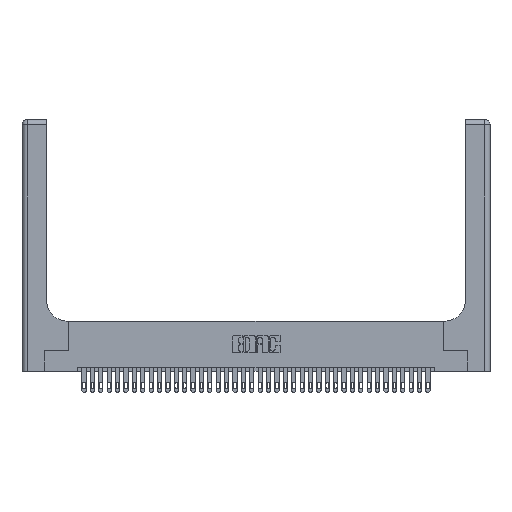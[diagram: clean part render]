
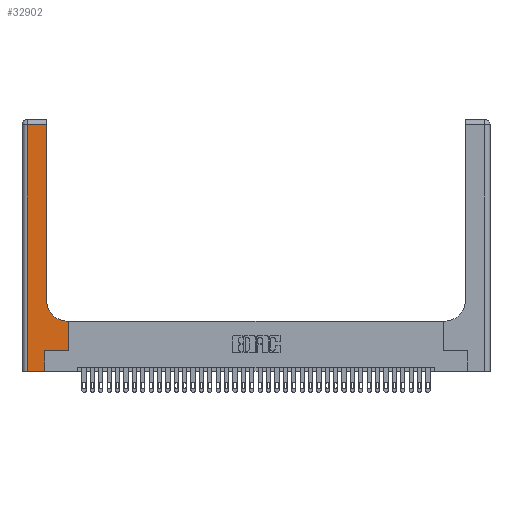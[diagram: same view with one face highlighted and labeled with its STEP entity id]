
A CAD part, top view. The second image highlights one B-rep face of the part: STEP entity #32902.
In plain terms, the highlighted planar face has unit normal (0, 0, 1).
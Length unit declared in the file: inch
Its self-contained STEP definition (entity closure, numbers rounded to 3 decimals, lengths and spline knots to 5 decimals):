
#487 = EDGE_CURVE ( 'NONE', #10428, #34353, #5170, .T. ) ;
#546 = CARTESIAN_POINT ( 'NONE',  ( 0.5585, 0.6, 0.37 ) ) ;
#2104 = CARTESIAN_POINT ( 'NONE',  ( 0.2915, 3., 0.37 ) ) ;
#2393 = ORIENTED_EDGE ( 'NONE', *, *, #11467, .T. ) ;
#2413 = CARTESIAN_POINT ( 'NONE',  ( 0.06, 3., 0.37 ) ) ;
#2970 = ORIENTED_EDGE ( 'NONE', *, *, #487, .T. ) ;
#3440 = VERTEX_POINT ( 'NONE', #29615 ) ;
#3580 = LINE ( 'NONE', #2104, #23335 ) ;
#5170 = LINE ( 'NONE', #30197, #10217 ) ;
#5419 = DIRECTION ( 'NONE',  ( -1., 0., 0. ) ) ;
#5505 = DIRECTION ( 'NONE',  ( -1., 0., 0. ) ) ;
#7911 = AXIS2_PLACEMENT_3D ( 'NONE', #28503, #28618, #5505 ) ;
#8545 = VECTOR ( 'NONE', #29272, 39.37008 ) ;
#9003 = ORIENTED_EDGE ( 'NONE', *, *, #17756, .T. ) ;
#9184 = DIRECTION ( 'NONE',  ( 1., 0., 0. ) ) ;
#9576 = ORIENTED_EDGE ( 'NONE', *, *, #9922, .T. ) ;
#9711 = EDGE_CURVE ( 'NONE', #27332, #13544, #22761, .T. ) ;
#9922 = EDGE_CURVE ( 'NONE', #34353, #3440, #23242, .T. ) ;
#10217 = VECTOR ( 'NONE', #21434, 39.37008 ) ;
#10428 = VERTEX_POINT ( 'NONE', #35386 ) ;
#10843 = VERTEX_POINT ( 'NONE', #28950 ) ;
#11359 = EDGE_CURVE ( 'NONE', #13544, #36346, #17511, .T. ) ;
#11467 = EDGE_CURVE ( 'NONE', #3440, #10843, #12934, .T. ) ;
#11985 = VERTEX_POINT ( 'NONE', #13174 ) ;
#12031 = VECTOR ( 'NONE', #14788, 39.37008 ) ;
#12079 = LINE ( 'NONE', #25442, #28228 ) ;
#12096 = ORIENTED_EDGE ( 'NONE', *, *, #37684, .T. ) ;
#12724 = ORIENTED_EDGE ( 'NONE', *, *, #9711, .T. ) ;
#12739 = CARTESIAN_POINT ( 'NONE',  ( 0.06, 2.94, 0.37 ) ) ;
#12934 = LINE ( 'NONE', #34843, #12031 ) ;
#13174 = CARTESIAN_POINT ( 'NONE',  ( 0.2915, 0.85, 0.37 ) ) ;
#13365 = EDGE_CURVE ( 'NONE', #11985, #10428, #3580, .T. ) ;
#13544 = VERTEX_POINT ( 'NONE', #546 ) ;
#14788 = DIRECTION ( 'NONE',  ( 1., 0., 0. ) ) ;
#17511 = LINE ( 'NONE', #29378, #19340 ) ;
#17756 = EDGE_CURVE ( 'NONE', #36346, #11985, #18513, .T. ) ;
#18512 = CARTESIAN_POINT ( 'NONE',  ( 0.269, 0.25, 0.37 ) ) ;
#18513 = CIRCLE ( 'NONE', #22358, 0.25 ) ;
#19340 = VECTOR ( 'NONE', #5419, 39.37008 ) ;
#19390 = LINE ( 'NONE', #18512, #28598 ) ;
#19884 = ORIENTED_EDGE ( 'NONE', *, *, #37550, .T. ) ;
#19935 = DIRECTION ( 'NONE',  ( 0., 1., 0. ) ) ;
#20149 = CARTESIAN_POINT ( 'NONE',  ( 0.5415, 0.6, 0.37 ) ) ;
#20582 = CARTESIAN_POINT ( 'NONE',  ( 0.5585, 0.25, 0.37 ) ) ;
#21181 = CARTESIAN_POINT ( 'NONE',  ( 0.269, 0.25, 0.37 ) ) ;
#21434 = DIRECTION ( 'NONE',  ( -1., 0., 0. ) ) ;
#21759 = ORIENTED_EDGE ( 'NONE', *, *, #13365, .T. ) ;
#21878 = FACE_OUTER_BOUND ( 'NONE', #36560, .T. ) ;
#22358 = AXIS2_PLACEMENT_3D ( 'NONE', #29987, #32949, #9184 ) ;
#22761 = LINE ( 'NONE', #23166, #30592 ) ;
#23166 = CARTESIAN_POINT ( 'NONE',  ( 0.5585, 0.25, 0.37 ) ) ;
#23242 = LINE ( 'NONE', #2413, #8545 ) ;
#23335 = VECTOR ( 'NONE', #19935, 39.37008 ) ;
#25442 = CARTESIAN_POINT ( 'NONE',  ( 0.269, 0., 0.37 ) ) ;
#27332 = VERTEX_POINT ( 'NONE', #20582 ) ;
#27481 = ORIENTED_EDGE ( 'NONE', *, *, #11359, .T. ) ;
#28096 = PLANE ( 'NONE',  #7911 ) ;
#28228 = VECTOR ( 'NONE', #31104, 39.37008 ) ;
#28503 = CARTESIAN_POINT ( 'NONE',  ( 0., 3., 0.37 ) ) ;
#28598 = VECTOR ( 'NONE', #30465, 39.37008 ) ;
#28618 = DIRECTION ( 'NONE',  ( 0., 0., -1. ) ) ;
#28846 = VERTEX_POINT ( 'NONE', #21181 ) ;
#28950 = CARTESIAN_POINT ( 'NONE',  ( 0.269, 0., 0.37 ) ) ;
#29114 = DIRECTION ( 'NONE',  ( 0., 1., 0. ) ) ;
#29272 = DIRECTION ( 'NONE',  ( 0., -1., 0. ) ) ;
#29378 = CARTESIAN_POINT ( 'NONE',  ( 0.2915, 0.6, 0.37 ) ) ;
#29615 = CARTESIAN_POINT ( 'NONE',  ( 0.06, 0., 0.37 ) ) ;
#29987 = CARTESIAN_POINT ( 'NONE',  ( 0.5415, 0.85, 0.37 ) ) ;
#30197 = CARTESIAN_POINT ( 'NONE',  ( 0., 2.94, 0.37 ) ) ;
#30465 = DIRECTION ( 'NONE',  ( 1., 0., 0. ) ) ;
#30592 = VECTOR ( 'NONE', #29114, 39.37008 ) ;
#31104 = DIRECTION ( 'NONE',  ( 0., 1., 0. ) ) ;
#32902 = ADVANCED_FACE ( 'NONE', ( #21878 ), #28096, .F. ) ;
#32949 = DIRECTION ( 'NONE',  ( 0., 0., -1. ) ) ;
#34353 = VERTEX_POINT ( 'NONE', #12739 ) ;
#34843 = CARTESIAN_POINT ( 'NONE',  ( 0., 0., 0.37 ) ) ;
#35386 = CARTESIAN_POINT ( 'NONE',  ( 0.2915, 2.94, 0.37 ) ) ;
#36346 = VERTEX_POINT ( 'NONE', #20149 ) ;
#36560 = EDGE_LOOP ( 'NONE', ( #21759, #2970, #9576, #2393, #12096, #19884, #12724, #27481, #9003 ) ) ;
#37550 = EDGE_CURVE ( 'NONE', #28846, #27332, #19390, .T. ) ;
#37684 = EDGE_CURVE ( 'NONE', #10843, #28846, #12079, .T. ) ;
